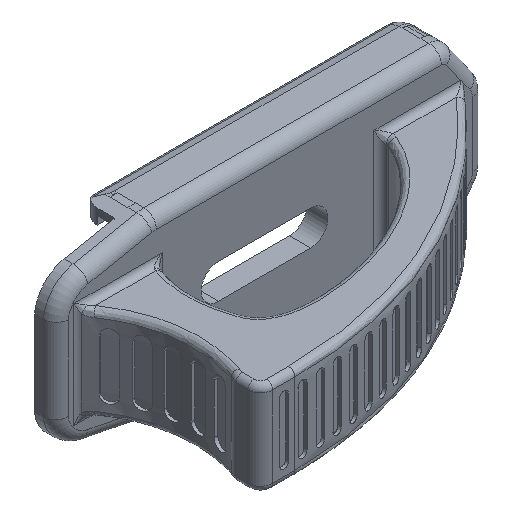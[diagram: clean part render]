
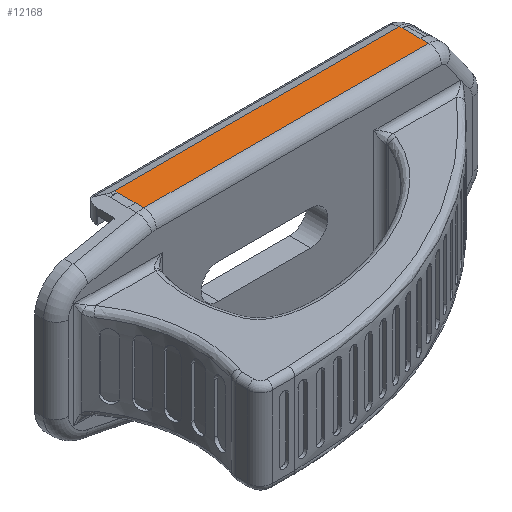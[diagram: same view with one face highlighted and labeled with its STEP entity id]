
A CAD part, isometric view. The second image highlights one B-rep face of the part: STEP entity #12168.
In plain terms, the highlighted face is planar.
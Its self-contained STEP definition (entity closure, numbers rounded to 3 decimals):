
#97 = VECTOR ( 'NONE', #18945, 1000. ) ;
#732 = LINE ( 'NONE', #9967, #2744 ) ;
#1116 = CARTESIAN_POINT ( 'NONE',  ( 14.2, -2.36, 7. ) ) ;
#1915 = ORIENTED_EDGE ( 'NONE', *, *, #5311, .T. ) ;
#2100 = EDGE_CURVE ( 'NONE', #15592, #18844, #10968, .T. ) ;
#2134 = DIRECTION ( 'NONE',  ( 0., -1., 0. ) ) ;
#2168 = VERTEX_POINT ( 'NONE', #15050 ) ;
#2375 = EDGE_LOOP ( 'NONE', ( #3403, #9112, #1915, #20350, #18708, #14964, #4206, #22788 ) ) ;
#2376 = LINE ( 'NONE', #13655, #3922 ) ;
#2523 = CARTESIAN_POINT ( 'NONE',  ( 14.2, -2.36, 7. ) ) ;
#2744 = VECTOR ( 'NONE', #17503, 1000. ) ;
#2776 = DIRECTION ( 'NONE',  ( -1., 0., 0. ) ) ;
#3009 = CARTESIAN_POINT ( 'NONE',  ( 14.2, -0.94, 52.748 ) ) ;
#3076 = AXIS2_PLACEMENT_3D ( 'NONE', #8177, #2776, #17273 ) ;
#3403 = ORIENTED_EDGE ( 'NONE', *, *, #8944, .F. ) ;
#3842 = VECTOR ( 'NONE', #19191, 1000. ) ;
#3922 = VECTOR ( 'NONE', #4418, 1000. ) ;
#4206 = ORIENTED_EDGE ( 'NONE', *, *, #2100, .F. ) ;
#4246 = CARTESIAN_POINT ( 'NONE',  ( 14.2, 1.91, 52.748 ) ) ;
#4418 = DIRECTION ( 'NONE',  ( 0., 0., 1. ) ) ;
#5311 = EDGE_CURVE ( 'NONE', #15728, #20477, #14155, .T. ) ;
#7411 = VECTOR ( 'NONE', #2134, 1000. ) ;
#8177 = CARTESIAN_POINT ( 'NONE',  ( 14.2, -0.94, 52.748 ) ) ;
#8411 = LINE ( 'NONE', #3009, #3842 ) ;
#8526 = PLANE ( 'NONE',  #3076 ) ;
#8944 = EDGE_CURVE ( 'NONE', #15054, #19197, #732, .T. ) ;
#9112 = ORIENTED_EDGE ( 'NONE', *, *, #13974, .T. ) ;
#9167 = DIRECTION ( 'NONE',  ( 0., -1., 0. ) ) ;
#9266 = VECTOR ( 'NONE', #10556, 1000. ) ;
#9967 = CARTESIAN_POINT ( 'NONE',  ( 14.2, 4.36, 7. ) ) ;
#10556 = DIRECTION ( 'NONE',  ( 0., -1., 0. ) ) ;
#10879 = CARTESIAN_POINT ( 'NONE',  ( 14.2, -2.36, 52.748 ) ) ;
#10968 = LINE ( 'NONE', #22115, #23584 ) ;
#11254 = CARTESIAN_POINT ( 'NONE',  ( 14.2, 1.91, 7. ) ) ;
#11370 = LINE ( 'NONE', #20110, #7411 ) ;
#11640 = LINE ( 'NONE', #2523, #97 ) ;
#12067 = EDGE_CURVE ( 'NONE', #2168, #22542, #8411, .T. ) ;
#12168 = ADVANCED_FACE ( 'NONE', ( #22796 ), #8526, .F. ) ;
#12646 = CARTESIAN_POINT ( 'NONE',  ( 14.2, 1.91, 52.748 ) ) ;
#12884 = LINE ( 'NONE', #12646, #15062 ) ;
#13655 = CARTESIAN_POINT ( 'NONE',  ( 14.2, 2.36, 52.748 ) ) ;
#13974 = EDGE_CURVE ( 'NONE', #15054, #15728, #2376, .T. ) ;
#14155 = LINE ( 'NONE', #18086, #9266 ) ;
#14964 = ORIENTED_EDGE ( 'NONE', *, *, #21703, .T. ) ;
#15050 = CARTESIAN_POINT ( 'NONE',  ( 14.2, -0.94, 52.748 ) ) ;
#15054 = VERTEX_POINT ( 'NONE', #22766 ) ;
#15062 = VECTOR ( 'NONE', #9167, 1000. ) ;
#15592 = VERTEX_POINT ( 'NONE', #23150 ) ;
#15728 = VERTEX_POINT ( 'NONE', #17863 ) ;
#16596 = EDGE_CURVE ( 'NONE', #20477, #2168, #12884, .T. ) ;
#17273 = DIRECTION ( 'NONE',  ( 0., 0., 1. ) ) ;
#17503 = DIRECTION ( 'NONE',  ( 0., -1., 0. ) ) ;
#17863 = CARTESIAN_POINT ( 'NONE',  ( 14.2, 2.36, 52.748 ) ) ;
#18086 = CARTESIAN_POINT ( 'NONE',  ( 14.2, 4.36, 52.748 ) ) ;
#18277 = DIRECTION ( 'NONE',  ( 0., -1., 0. ) ) ;
#18708 = ORIENTED_EDGE ( 'NONE', *, *, #12067, .T. ) ;
#18844 = VERTEX_POINT ( 'NONE', #1116 ) ;
#18945 = DIRECTION ( 'NONE',  ( 0., 0., -1. ) ) ;
#19191 = DIRECTION ( 'NONE',  ( 0., -1., 0. ) ) ;
#19197 = VERTEX_POINT ( 'NONE', #11254 ) ;
#19236 = EDGE_CURVE ( 'NONE', #19197, #15592, #11370, .T. ) ;
#20110 = CARTESIAN_POINT ( 'NONE',  ( 14.2, 1.91, 7. ) ) ;
#20350 = ORIENTED_EDGE ( 'NONE', *, *, #16596, .T. ) ;
#20477 = VERTEX_POINT ( 'NONE', #4246 ) ;
#21703 = EDGE_CURVE ( 'NONE', #22542, #18844, #11640, .T. ) ;
#22115 = CARTESIAN_POINT ( 'NONE',  ( 14.2, -0.94, 7. ) ) ;
#22542 = VERTEX_POINT ( 'NONE', #10879 ) ;
#22766 = CARTESIAN_POINT ( 'NONE',  ( 14.2, 2.36, 7. ) ) ;
#22788 = ORIENTED_EDGE ( 'NONE', *, *, #19236, .F. ) ;
#22796 = FACE_OUTER_BOUND ( 'NONE', #2375, .T. ) ;
#23150 = CARTESIAN_POINT ( 'NONE',  ( 14.2, -0.94, 7. ) ) ;
#23584 = VECTOR ( 'NONE', #18277, 1000. ) ;
